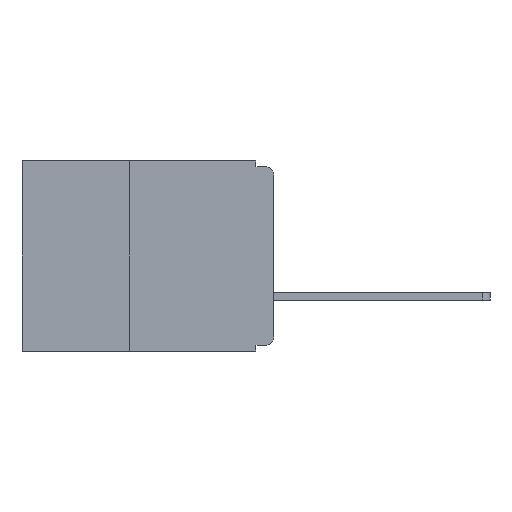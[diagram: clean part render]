
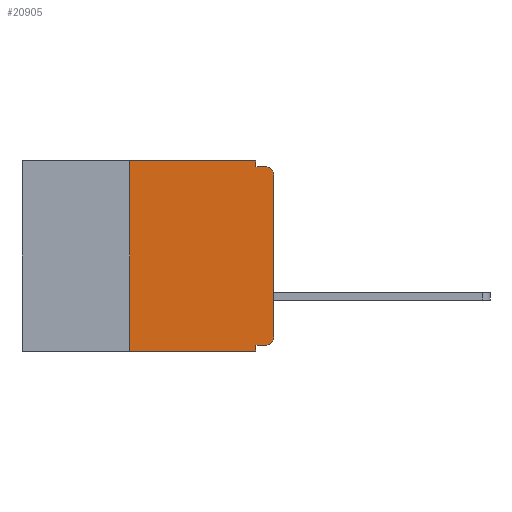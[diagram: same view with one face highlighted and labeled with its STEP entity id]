
A CAD part, left-side view. The second image highlights one B-rep face of the part: STEP entity #20905.
In plain terms, the highlighted planar face has unit normal (-1, 0, 0).
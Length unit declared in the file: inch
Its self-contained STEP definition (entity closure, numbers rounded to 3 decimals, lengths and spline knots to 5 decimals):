
#283 = VERTEX_POINT ( 'NONE', #20115 ) ;
#1510 = ORIENTED_EDGE ( 'NONE', *, *, #29227, .F. ) ;
#1988 = CARTESIAN_POINT ( 'NONE',  ( 0., 0.25, -0.33 ) ) ;
#2093 = EDGE_CURVE ( 'NONE', #17406, #20787, #6973, .T. ) ;
#2342 = LINE ( 'NONE', #12416, #21272 ) ;
#3228 = VERTEX_POINT ( 'NONE', #7930 ) ;
#3447 = CARTESIAN_POINT ( 'NONE',  ( 0., 0.031, -0.01 ) ) ;
#3465 = CARTESIAN_POINT ( 'NONE',  ( 0., 0.015, -0.01 ) ) ;
#3681 = EDGE_CURVE ( 'NONE', #3228, #17406, #2342, .T. ) ;
#4100 = EDGE_CURVE ( 'NONE', #17204, #31297, #22816, .T. ) ;
#4869 = VECTOR ( 'NONE', #32245, 39.37008 ) ;
#5543 = VERTEX_POINT ( 'NONE', #18268 ) ;
#5676 = CARTESIAN_POINT ( 'NONE',  ( 0., 0.031, 0. ) ) ;
#5734 = VECTOR ( 'NONE', #19381, 39.37008 ) ;
#6067 = CARTESIAN_POINT ( 'NONE',  ( 0., 0.015, -0.025 ) ) ;
#6367 = LINE ( 'NONE', #7752, #32702 ) ;
#6726 = CARTESIAN_POINT ( 'NONE',  ( 0., 0.031, -0.32 ) ) ;
#6973 = LINE ( 'NONE', #5676, #31718 ) ;
#7069 = AXIS2_PLACEMENT_3D ( 'NONE', #14387, #32159, #16950 ) ;
#7611 = ORIENTED_EDGE ( 'NONE', *, *, #23683, .F. ) ;
#7752 = CARTESIAN_POINT ( 'NONE',  ( 0., 0.437, -0.33 ) ) ;
#7930 = CARTESIAN_POINT ( 'NONE',  ( 0., 0.25, 0. ) ) ;
#8003 = ORIENTED_EDGE ( 'NONE', *, *, #14713, .T. ) ;
#8676 = DIRECTION ( 'NONE',  ( 0., 0., -1. ) ) ;
#8693 = AXIS2_PLACEMENT_3D ( 'NONE', #6067, #23987, #8676 ) ;
#10921 = VERTEX_POINT ( 'NONE', #6726 ) ;
#11792 = PLANE ( 'NONE',  #7069 ) ;
#11993 = CARTESIAN_POINT ( 'NONE',  ( 0., 0., -0.01 ) ) ;
#12416 = CARTESIAN_POINT ( 'NONE',  ( 0., 0.437, 0. ) ) ;
#12473 = ORIENTED_EDGE ( 'NONE', *, *, #19028, .T. ) ;
#13488 = FACE_OUTER_BOUND ( 'NONE', #18736, .T. ) ;
#14387 = CARTESIAN_POINT ( 'NONE',  ( 0., 0.437, 0. ) ) ;
#14398 = AXIS2_PLACEMENT_3D ( 'NONE', #30088, #30046, #29070 ) ;
#14458 = CARTESIAN_POINT ( 'NONE',  ( 0., 0.031, 0. ) ) ;
#14713 = EDGE_CURVE ( 'NONE', #31297, #5543, #21079, .T. ) ;
#14818 = DIRECTION ( 'NONE',  ( 0., 0., -1. ) ) ;
#14862 = ORIENTED_EDGE ( 'NONE', *, *, #3681, .F. ) ;
#15352 = ORIENTED_EDGE ( 'NONE', *, *, #4100, .T. ) ;
#16005 = VECTOR ( 'NONE', #16195, 39.37008 ) ;
#16195 = DIRECTION ( 'NONE',  ( 0., 0., -1. ) ) ;
#16545 = EDGE_CURVE ( 'NONE', #5543, #32832, #30091, .T. ) ;
#16848 = ORIENTED_EDGE ( 'NONE', *, *, #2093, .F. ) ;
#16950 = DIRECTION ( 'NONE',  ( 0., 0., -1. ) ) ;
#17204 = VERTEX_POINT ( 'NONE', #26413 ) ;
#17406 = VERTEX_POINT ( 'NONE', #14458 ) ;
#18268 = CARTESIAN_POINT ( 'NONE',  ( 0., 0., -0.025 ) ) ;
#18736 = EDGE_LOOP ( 'NONE', ( #8003, #30773, #7611, #16848, #14862, #1510, #12473, #24070, #19312, #15352 ) ) ;
#19028 = EDGE_CURVE ( 'NONE', #22581, #283, #6367, .T. ) ;
#19094 = CARTESIAN_POINT ( 'NONE',  ( 0., 0.25, -0.33 ) ) ;
#19312 = ORIENTED_EDGE ( 'NONE', *, *, #23266, .F. ) ;
#19356 = LINE ( 'NONE', #11993, #4869 ) ;
#19363 = VECTOR ( 'NONE', #22566, 39.37008 ) ;
#19381 = DIRECTION ( 'NONE',  ( 0., 1., 0. ) ) ;
#20115 = CARTESIAN_POINT ( 'NONE',  ( 0., 0.031, -0.33 ) ) ;
#20571 = DIRECTION ( 'NONE',  ( 0., 0., 1. ) ) ;
#20787 = VERTEX_POINT ( 'NONE', #3447 ) ;
#20905 = ADVANCED_FACE ( 'NONE', ( #13488 ), #11792, .F. ) ;
#21079 = LINE ( 'NONE', #28157, #26274 ) ;
#21272 = VECTOR ( 'NONE', #31872, 39.37008 ) ;
#22036 = CARTESIAN_POINT ( 'NONE',  ( 0., 0., -0.32 ) ) ;
#22566 = DIRECTION ( 'NONE',  ( 0., 0., 1. ) ) ;
#22581 = VERTEX_POINT ( 'NONE', #19094 ) ;
#22764 = LINE ( 'NONE', #31422, #16005 ) ;
#22816 = CIRCLE ( 'NONE', #14398, 0.015 ) ;
#23068 = DIRECTION ( 'NONE',  ( 0., -1., 0. ) ) ;
#23266 = EDGE_CURVE ( 'NONE', #17204, #10921, #25375, .T. ) ;
#23683 = EDGE_CURVE ( 'NONE', #20787, #32832, #19356, .T. ) ;
#23987 = DIRECTION ( 'NONE',  ( -1., 0., 0. ) ) ;
#24070 = ORIENTED_EDGE ( 'NONE', *, *, #26557, .F. ) ;
#25375 = LINE ( 'NONE', #22036, #5734 ) ;
#26274 = VECTOR ( 'NONE', #20571, 39.37008 ) ;
#26413 = CARTESIAN_POINT ( 'NONE',  ( 0., 0.015, -0.32 ) ) ;
#26557 = EDGE_CURVE ( 'NONE', #10921, #283, #22764, .T. ) ;
#26926 = LINE ( 'NONE', #1988, #19363 ) ;
#28157 = CARTESIAN_POINT ( 'NONE',  ( 0., 0., 0. ) ) ;
#29070 = DIRECTION ( 'NONE',  ( 0., 0., -1. ) ) ;
#29227 = EDGE_CURVE ( 'NONE', #22581, #3228, #26926, .T. ) ;
#30046 = DIRECTION ( 'NONE',  ( -1., 0., 0. ) ) ;
#30088 = CARTESIAN_POINT ( 'NONE',  ( 0., 0.015, -0.305 ) ) ;
#30091 = CIRCLE ( 'NONE', #8693, 0.015 ) ;
#30773 = ORIENTED_EDGE ( 'NONE', *, *, #16545, .T. ) ;
#31297 = VERTEX_POINT ( 'NONE', #31552 ) ;
#31422 = CARTESIAN_POINT ( 'NONE',  ( 0., 0.031, -0.33 ) ) ;
#31552 = CARTESIAN_POINT ( 'NONE',  ( 0., 0., -0.305 ) ) ;
#31718 = VECTOR ( 'NONE', #14818, 39.37008 ) ;
#31872 = DIRECTION ( 'NONE',  ( 0., -1., 0. ) ) ;
#32159 = DIRECTION ( 'NONE',  ( 1., 0., 0. ) ) ;
#32245 = DIRECTION ( 'NONE',  ( 0., -1., 0. ) ) ;
#32702 = VECTOR ( 'NONE', #23068, 39.37008 ) ;
#32832 = VERTEX_POINT ( 'NONE', #3465 ) ;
